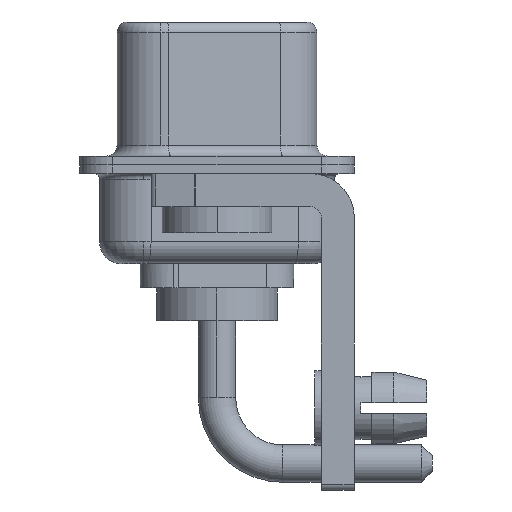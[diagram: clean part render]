
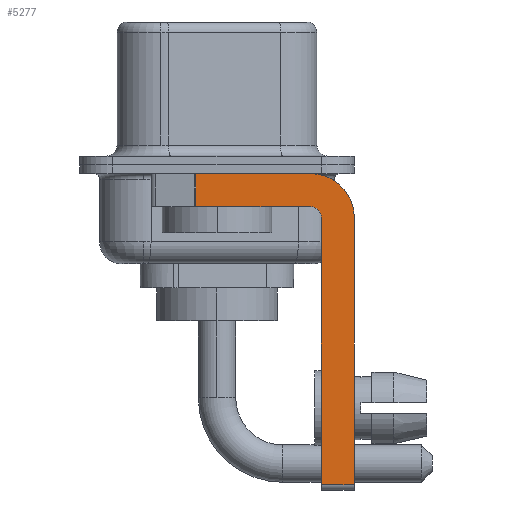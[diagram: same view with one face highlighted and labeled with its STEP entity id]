
A CAD part, left-side view. The second image highlights one B-rep face of the part: STEP entity #5277.
In plain terms, the highlighted planar face has unit normal (-1, 0, 0).
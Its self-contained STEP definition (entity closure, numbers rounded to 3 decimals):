
#26 = DIRECTION ( 'NONE',  ( 0., 0., -1. ) ) ;
#348 = LINE ( 'NONE', #16344, #8963 ) ;
#656 = VERTEX_POINT ( 'NONE', #2766 ) ;
#894 = CARTESIAN_POINT ( 'NONE',  ( -2.9, 0.978, -1.9 ) ) ;
#1181 = CIRCLE ( 'NONE', #9925, 0.5 ) ;
#1317 = DIRECTION ( 'NONE',  ( 1., 0., 0. ) ) ;
#1352 = LINE ( 'NONE', #15130, #11373 ) ;
#1588 = VERTEX_POINT ( 'NONE', #13678 ) ;
#2034 = EDGE_CURVE ( 'NONE', #12155, #5600, #5606, .T. ) ;
#2156 = LINE ( 'NONE', #12352, #16354 ) ;
#2488 = VERTEX_POINT ( 'NONE', #13045 ) ;
#2746 = LINE ( 'NONE', #5763, #3399 ) ;
#2766 = CARTESIAN_POINT ( 'NONE',  ( -2.9, -4.25, -0.4 ) ) ;
#3352 = ORIENTED_EDGE ( 'NONE', *, *, #12458, .F. ) ;
#3383 = ORIENTED_EDGE ( 'NONE', *, *, #2034, .F. ) ;
#3399 = VECTOR ( 'NONE', #8207, 1000. ) ;
#4030 = ORIENTED_EDGE ( 'NONE', *, *, #10755, .F. ) ;
#4104 = EDGE_CURVE ( 'NONE', #8126, #8204, #2156, .T. ) ;
#4412 = CARTESIAN_POINT ( 'NONE',  ( -2.9, 0.978, -0.4 ) ) ;
#4573 = CARTESIAN_POINT ( 'NONE',  ( -2.9, -4.75, -14.8 ) ) ;
#5186 = DIRECTION ( 'NONE',  ( -1., 0., 0. ) ) ;
#5195 = CARTESIAN_POINT ( 'NONE',  ( -2.9, -6.25, -2.4 ) ) ;
#5277 = ADVANCED_FACE ( 'NONE', ( #7888 ), #13144, .F. ) ;
#5600 = VERTEX_POINT ( 'NONE', #15522 ) ;
#5606 = LINE ( 'NONE', #7984, #14803 ) ;
#5763 = CARTESIAN_POINT ( 'NONE',  ( -2.9, -4.25, -1.9 ) ) ;
#7026 = DIRECTION ( 'NONE',  ( 0., 0., -1. ) ) ;
#7836 = EDGE_CURVE ( 'NONE', #2488, #1588, #1181, .T. ) ;
#7888 = FACE_OUTER_BOUND ( 'NONE', #11520, .T. ) ;
#7984 = CARTESIAN_POINT ( 'NONE',  ( -2.9, -6.25, -2.4 ) ) ;
#8126 = VERTEX_POINT ( 'NONE', #4412 ) ;
#8204 = VERTEX_POINT ( 'NONE', #894 ) ;
#8207 = DIRECTION ( 'NONE',  ( 0., 1., 0. ) ) ;
#8585 = ORIENTED_EDGE ( 'NONE', *, *, #4104, .T. ) ;
#8963 = VECTOR ( 'NONE', #9811, 1000. ) ;
#9124 = DIRECTION ( 'NONE',  ( 0., 0., 1. ) ) ;
#9471 = AXIS2_PLACEMENT_3D ( 'NONE', #13512, #16340, #12308 ) ;
#9549 = DIRECTION ( 'NONE',  ( 0., 0., -1. ) ) ;
#9608 = EDGE_CURVE ( 'NONE', #15034, #2488, #15210, .T. ) ;
#9643 = DIRECTION ( 'NONE',  ( 0., -1., 0. ) ) ;
#9720 = DIRECTION ( 'NONE',  ( 0., 0., 1. ) ) ;
#9811 = DIRECTION ( 'NONE',  ( 0., -1., 0. ) ) ;
#9925 = AXIS2_PLACEMENT_3D ( 'NONE', #12901, #5186, #9124 ) ;
#10755 = EDGE_CURVE ( 'NONE', #1588, #8204, #2746, .T. ) ;
#11373 = VECTOR ( 'NONE', #9643, 1000. ) ;
#11478 = ORIENTED_EDGE ( 'NONE', *, *, #7836, .F. ) ;
#11520 = EDGE_LOOP ( 'NONE', ( #13974, #8585, #4030, #11478, #11575, #15520, #3383, #3352 ) ) ;
#11575 = ORIENTED_EDGE ( 'NONE', *, *, #9608, .F. ) ;
#12155 = VERTEX_POINT ( 'NONE', #5195 ) ;
#12308 = DIRECTION ( 'NONE',  ( 0., 0., -1. ) ) ;
#12352 = CARTESIAN_POINT ( 'NONE',  ( -2.9, 0.978, -1.9 ) ) ;
#12365 = EDGE_CURVE ( 'NONE', #15034, #5600, #1352, .T. ) ;
#12458 = EDGE_CURVE ( 'NONE', #656, #12155, #16874, .T. ) ;
#12901 = CARTESIAN_POINT ( 'NONE',  ( -2.9, -4.25, -2.4 ) ) ;
#13045 = CARTESIAN_POINT ( 'NONE',  ( -2.9, -4.75, -2.4 ) ) ;
#13050 = CARTESIAN_POINT ( 'NONE',  ( -2.9, -4.25, -2.4 ) ) ;
#13144 = PLANE ( 'NONE',  #16805 ) ;
#13512 = CARTESIAN_POINT ( 'NONE',  ( -2.9, -4.25, -2.4 ) ) ;
#13678 = CARTESIAN_POINT ( 'NONE',  ( -2.9, -4.25, -1.9 ) ) ;
#13974 = ORIENTED_EDGE ( 'NONE', *, *, #15023, .F. ) ;
#14803 = VECTOR ( 'NONE', #9549, 1000. ) ;
#15023 = EDGE_CURVE ( 'NONE', #8126, #656, #348, .T. ) ;
#15034 = VERTEX_POINT ( 'NONE', #16429 ) ;
#15130 = CARTESIAN_POINT ( 'NONE',  ( -2.9, -4.25, -14.55 ) ) ;
#15138 = VECTOR ( 'NONE', #9720, 1000. ) ;
#15210 = LINE ( 'NONE', #4573, #15138 ) ;
#15520 = ORIENTED_EDGE ( 'NONE', *, *, #12365, .T. ) ;
#15522 = CARTESIAN_POINT ( 'NONE',  ( -2.9, -6.25, -14.55 ) ) ;
#16340 = DIRECTION ( 'NONE',  ( 1., 0., 0. ) ) ;
#16344 = CARTESIAN_POINT ( 'NONE',  ( -2.9, 3., -0.4 ) ) ;
#16354 = VECTOR ( 'NONE', #7026, 1000. ) ;
#16429 = CARTESIAN_POINT ( 'NONE',  ( -2.9, -4.75, -14.55 ) ) ;
#16805 = AXIS2_PLACEMENT_3D ( 'NONE', #13050, #1317, #26 ) ;
#16874 = CIRCLE ( 'NONE', #9471, 2. ) ;
